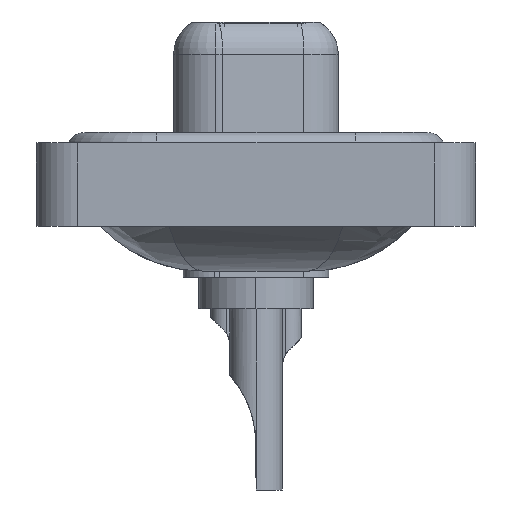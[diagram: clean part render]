
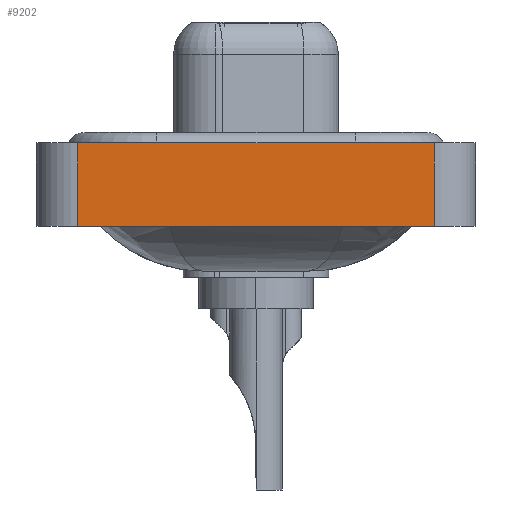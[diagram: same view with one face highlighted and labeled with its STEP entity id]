
A CAD part, left-side view. The second image highlights one B-rep face of the part: STEP entity #9202.
In plain terms, the highlighted planar face has unit normal (-1, 0, 0).
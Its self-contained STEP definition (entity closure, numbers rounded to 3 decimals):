
#305 = DIRECTION ( 'NONE',  ( 0., -1., 0. ) ) ;
#475 = CARTESIAN_POINT ( 'NONE',  ( -7.35, 8.55, 0.4 ) ) ;
#688 = EDGE_CURVE ( 'NONE', #5812, #13465, #12566, .T. ) ;
#1130 = DIRECTION ( 'NONE',  ( 0., 0., 1. ) ) ;
#1441 = VECTOR ( 'NONE', #14718, 1000. ) ;
#1990 = ORIENTED_EDGE ( 'NONE', *, *, #9552, .F. ) ;
#3109 = DIRECTION ( 'NONE',  ( 0., 0., 1. ) ) ;
#3267 = DIRECTION ( 'NONE',  ( -1., 0., 0. ) ) ;
#3401 = CARTESIAN_POINT ( 'NONE',  ( -7.35, 8.55, -3.6 ) ) ;
#3754 = ORIENTED_EDGE ( 'NONE', *, *, #13683, .T. ) ;
#5011 = ORIENTED_EDGE ( 'NONE', *, *, #688, .T. ) ;
#5812 = VERTEX_POINT ( 'NONE', #18003 ) ;
#8050 = EDGE_LOOP ( 'NONE', ( #5011, #10827, #1990, #3754 ) ) ;
#9202 = ADVANCED_FACE ( 'NONE', ( #24315 ), #22422, .T. ) ;
#9450 = VERTEX_POINT ( 'NONE', #475 ) ;
#9552 = EDGE_CURVE ( 'NONE', #13595, #9450, #10556, .T. ) ;
#10556 = LINE ( 'NONE', #18377, #1441 ) ;
#10683 = CARTESIAN_POINT ( 'NONE',  ( -7.35, -8.55, -3.6 ) ) ;
#10827 = ORIENTED_EDGE ( 'NONE', *, *, #16425, .F. ) ;
#11529 = CARTESIAN_POINT ( 'NONE',  ( -7.35, -8.55, 0.4 ) ) ;
#12488 = CARTESIAN_POINT ( 'NONE',  ( -7.35, -8.55, 0.4 ) ) ;
#12566 = LINE ( 'NONE', #10683, #19896 ) ;
#13242 = CARTESIAN_POINT ( 'NONE',  ( -7.35, -8.55, -3.6 ) ) ;
#13465 = VERTEX_POINT ( 'NONE', #12488 ) ;
#13509 = AXIS2_PLACEMENT_3D ( 'NONE', #14504, #3267, #1130 ) ;
#13595 = VERTEX_POINT ( 'NONE', #3401 ) ;
#13683 = EDGE_CURVE ( 'NONE', #13595, #5812, #17149, .T. ) ;
#14504 = CARTESIAN_POINT ( 'NONE',  ( -7.35, -8.55, -3.6 ) ) ;
#14718 = DIRECTION ( 'NONE',  ( 0., 0., 1. ) ) ;
#16425 = EDGE_CURVE ( 'NONE', #9450, #13465, #19726, .T. ) ;
#17149 = LINE ( 'NONE', #13242, #24083 ) ;
#18003 = CARTESIAN_POINT ( 'NONE',  ( -7.35, -8.55, -3.6 ) ) ;
#18377 = CARTESIAN_POINT ( 'NONE',  ( -7.35, 8.55, -3.6 ) ) ;
#19726 = LINE ( 'NONE', #11529, #22644 ) ;
#19896 = VECTOR ( 'NONE', #3109, 1000. ) ;
#22422 = PLANE ( 'NONE',  #13509 ) ;
#22644 = VECTOR ( 'NONE', #305, 1000. ) ;
#24083 = VECTOR ( 'NONE', #24832, 1000. ) ;
#24315 = FACE_OUTER_BOUND ( 'NONE', #8050, .T. ) ;
#24832 = DIRECTION ( 'NONE',  ( 0., -1., 0. ) ) ;
